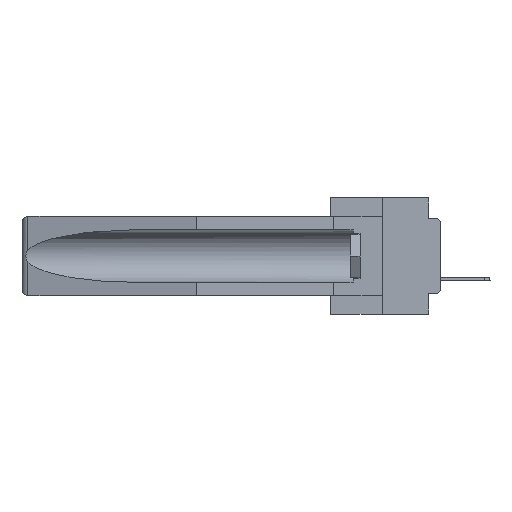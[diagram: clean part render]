
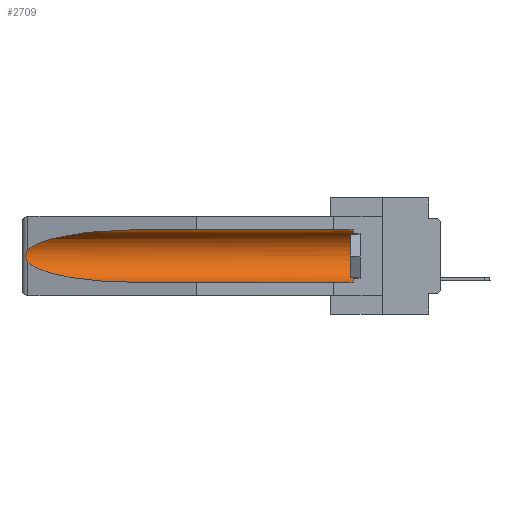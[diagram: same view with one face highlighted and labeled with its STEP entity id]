
A CAD part, left-side view. The second image highlights one B-rep face of the part: STEP entity #2709.
In plain terms, the highlighted cylindrical face has radius 2.857 mm (diameter 5.715 mm), a partial arc.
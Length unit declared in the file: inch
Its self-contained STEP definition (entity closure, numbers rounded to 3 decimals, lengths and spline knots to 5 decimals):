
#661 = DIRECTION ( 'NONE',  ( 0., 0., 1. ) ) ;
#1881 = B_SPLINE_CURVE_WITH_KNOTS ( 'NONE', 3,
 ( #9354, #27678, #7112, #11758, #29343, #27073, #4266, #8910, #16427, #27980 ),
 .UNSPECIFIED., .F., .F.,
 ( 4, 2, 2, 2, 4 ),
 ( 0., 0.00029, 0.00058, 0.00087, 0.00117 ),
 .UNSPECIFIED. ) ;
#1963 = EDGE_CURVE ( 'NONE', #24866, #20283, #12975, .T. ) ;
#2392 = LINE ( 'NONE', #5222, #23707 ) ;
#2709 = ADVANCED_FACE ( 'NONE', ( #23463 ), #7524, .F. ) ;
#2915 = ORIENTED_EDGE ( 'NONE', *, *, #19058, .T. ) ;
#4266 = CARTESIAN_POINT ( 'NONE',  ( 0.2673, 1.53269, -0.17917 ) ) ;
#4554 = CARTESIAN_POINT ( 'NONE',  ( 0.155, 1.07973, -0.284 ) ) ;
#4681 = CARTESIAN_POINT ( 'NONE',  ( 0.26537, 1.52718, -0.19328 ) ) ;
#4831 = CARTESIAN_POINT ( 'NONE',  ( 0.155, 1.07973, -0.284 ) ) ;
#5158 = EDGE_CURVE ( 'NONE', #13391, #20283, #22206, .T. ) ;
#5222 = CARTESIAN_POINT ( 'NONE',  ( 0.155, -0.30754, -0.059 ) ) ;
#7112 = CARTESIAN_POINT ( 'NONE',  ( 0.26654, 1.53092, -0.15636 ) ) ;
#7524 = CYLINDRICAL_SURFACE ( 'NONE', #27050, 0.1125 ) ;
#7847 = EDGE_CURVE ( 'NONE', #20368, #24002, #25062, .T. ) ;
#8910 = CARTESIAN_POINT ( 'NONE',  ( 0.26655, 1.53094, -0.18657 ) ) ;
#9354 = CARTESIAN_POINT ( 'NONE',  ( 0.26537, 1.52718, -0.14972 ) ) ;
#10236 = CARTESIAN_POINT ( 'NONE',  ( 0.26537, 1.52718, -0.14972 ) ) ;
#11281 = ORIENTED_EDGE ( 'NONE', *, *, #5158, .T. ) ;
#11620 = EDGE_LOOP ( 'NONE', ( #12726, #21853, #11281, #27009, #2915, #16151 ) ) ;
#11758 = CARTESIAN_POINT ( 'NONE',  ( 0.2673, 1.5327, -0.16383 ) ) ;
#12023 = CARTESIAN_POINT ( 'NONE',  ( 0.155, -0.30754, -0.1715 ) ) ;
#12726 = ORIENTED_EDGE ( 'NONE', *, *, #7847, .T. ) ;
#12851 = CARTESIAN_POINT ( 'NONE',  ( 0.26537, 1.52718, -0.14972 ) ) ;
#12975 = LINE ( 'NONE', #29205, #17434 ) ;
#13131 = EDGE_CURVE ( 'NONE', #24002, #13391, #1881, .T. ) ;
#13391 = VERTEX_POINT ( 'NONE', #4681 ) ;
#14152 = CARTESIAN_POINT ( 'NONE',  ( 0.26537, 1.52718, -0.19328 ) ) ;
#14224 = DIRECTION ( 'NONE',  ( 0., 1., 0. ) ) ;
#15953 = CARTESIAN_POINT ( 'NONE',  ( 0.21114, 1.30732, -0.284 ) ) ;
#16151 = ORIENTED_EDGE ( 'NONE', *, *, #21243, .T. ) ;
#16427 = CARTESIAN_POINT ( 'NONE',  ( 0.26597, 1.5296, -0.19026 ) ) ;
#17251 = CARTESIAN_POINT ( 'NONE',  ( 0.155, 0.126, -0.1715 ) ) ;
#17434 = VECTOR ( 'NONE', #26642, 39.37008 ) ;
#17692 = AXIS2_PLACEMENT_3D ( 'NONE', #17251, #21769, #26542 ) ;
#18718 = CARTESIAN_POINT ( 'NONE',  ( 0.21114, 1.30732, -0.059 ) ) ;
#18928 = CARTESIAN_POINT ( 'NONE',  ( 0.155, 1.07973, -0.059 ) ) ;
#19058 = EDGE_CURVE ( 'NONE', #24866, #29172, #21539, .T. ) ;
#19097 = DIRECTION ( 'NONE',  ( 0., 1., 0. ) ) ;
#20283 = VERTEX_POINT ( 'NONE', #4831 ) ;
#20368 = VERTEX_POINT ( 'NONE', #18928 ) ;
#20438 = CARTESIAN_POINT ( 'NONE',  ( 0.155, 0.126, -0.284 ) ) ;
#21243 = EDGE_CURVE ( 'NONE', #29172, #20368, #2392, .T. ) ;
#21539 = CIRCLE ( 'NONE', #17692, 0.1125 ) ;
#21769 = DIRECTION ( 'NONE',  ( 0., -1., 0. ) ) ;
#21824 = CARTESIAN_POINT ( 'NONE',  ( 0.155, 1.07973, -0.059 ) ) ;
#21853 = ORIENTED_EDGE ( 'NONE', *, *, #13131, .T. ) ;
#22206 =( BOUNDED_CURVE ( )  B_SPLINE_CURVE ( 3, ( #14152, #25421, #15953, #4554 ),
 .UNSPECIFIED., .F., .F. ) 
 B_SPLINE_CURVE_WITH_KNOTS ( ( 4, 4 ),
 ( 0.1948, 1.5708 ),
 .UNSPECIFIED. ) 
 CURVE ( )  GEOMETRIC_REPRESENTATION_ITEM ( )  RATIONAL_B_SPLINE_CURVE ( ( 1., 0.848, 0.848, 1. ) ) 
 REPRESENTATION_ITEM ( '' )  );
#23463 = FACE_OUTER_BOUND ( 'NONE', #11620, .T. ) ;
#23707 = VECTOR ( 'NONE', #14224, 39.37008 ) ;
#24002 = VERTEX_POINT ( 'NONE', #12851 ) ;
#24866 = VERTEX_POINT ( 'NONE', #20438 ) ;
#25062 =( BOUNDED_CURVE ( )  B_SPLINE_CURVE ( 3, ( #21824, #18718, #27876, #10236 ),
 .UNSPECIFIED., .F., .F. ) 
 B_SPLINE_CURVE_WITH_KNOTS ( ( 4, 4 ),
 ( 4.71239, 6.08839 ),
 .UNSPECIFIED. ) 
 CURVE ( )  GEOMETRIC_REPRESENTATION_ITEM ( )  RATIONAL_B_SPLINE_CURVE ( ( 1., 0.848, 0.848, 1. ) ) 
 REPRESENTATION_ITEM ( '' )  );
#25421 = CARTESIAN_POINT ( 'NONE',  ( 0.25451, 1.48313, -0.24835 ) ) ;
#25589 = CARTESIAN_POINT ( 'NONE',  ( 0.155, 0.126, -0.059 ) ) ;
#26542 = DIRECTION ( 'NONE',  ( 0., 0., 1. ) ) ;
#26642 = DIRECTION ( 'NONE',  ( 0., 1., 0. ) ) ;
#27009 = ORIENTED_EDGE ( 'NONE', *, *, #1963, .F. ) ;
#27050 = AXIS2_PLACEMENT_3D ( 'NONE', #12023, #19097, #661 ) ;
#27073 = CARTESIAN_POINT ( 'NONE',  ( 0.2675, 1.53308, -0.17534 ) ) ;
#27678 = CARTESIAN_POINT ( 'NONE',  ( 0.26597, 1.52961, -0.15275 ) ) ;
#27876 = CARTESIAN_POINT ( 'NONE',  ( 0.25451, 1.48313, -0.09465 ) ) ;
#27980 = CARTESIAN_POINT ( 'NONE',  ( 0.26537, 1.52718, -0.19328 ) ) ;
#29172 = VERTEX_POINT ( 'NONE', #25589 ) ;
#29205 = CARTESIAN_POINT ( 'NONE',  ( 0.155, -0.30754, -0.284 ) ) ;
#29343 = CARTESIAN_POINT ( 'NONE',  ( 0.2675, 1.53308, -0.16763 ) ) ;
